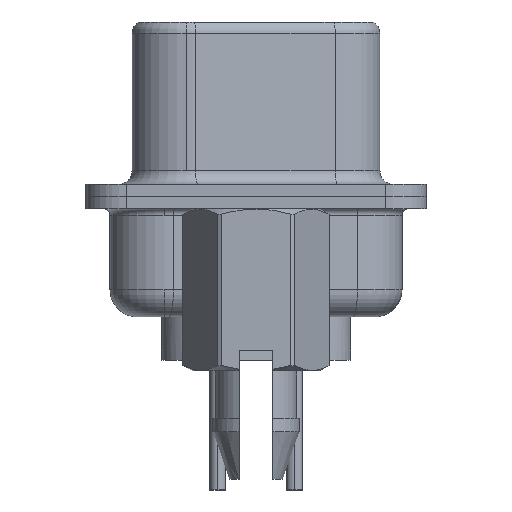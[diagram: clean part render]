
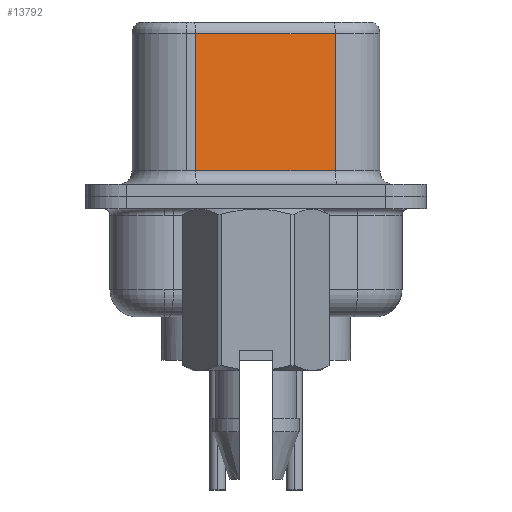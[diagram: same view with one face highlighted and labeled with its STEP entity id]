
A CAD part, left-side view. The second image highlights one B-rep face of the part: STEP entity #13792.
In plain terms, the highlighted planar face has unit normal (-0.985, -0.174, 0).
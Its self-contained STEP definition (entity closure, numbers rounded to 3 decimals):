
#142 = EDGE_CURVE ( 'NONE', #10876, #19702, #15350, .T. ) ;
#304 = LINE ( 'NONE', #4897, #16379 ) ;
#323 = VERTEX_POINT ( 'NONE', #346 ) ;
#346 = CARTESIAN_POINT ( 'NONE',  ( 4.575, -2.927, 6.02 ) ) ;
#371 = ORIENTED_EDGE ( 'NONE', *, *, #2547, .T. ) ;
#409 = DIRECTION ( 'NONE',  ( -0.174, 0.985, 0. ) ) ;
#1336 = ORIENTED_EDGE ( 'NONE', *, *, #4125, .T. ) ;
#1759 = CARTESIAN_POINT ( 'NONE',  ( 3.665, 2.233, 6.52 ) ) ;
#2231 = DIRECTION ( 'NONE',  ( 0.985, 0.174, 0. ) ) ;
#2373 = LINE ( 'NONE', #5272, #3210 ) ;
#2429 = PLANE ( 'NONE',  #13320 ) ;
#2547 = EDGE_CURVE ( 'NONE', #323, #10876, #304, .T. ) ;
#3210 = VECTOR ( 'NONE', #13266, 1000. ) ;
#3306 = VECTOR ( 'NONE', #12188, 1000. ) ;
#4047 = ORIENTED_EDGE ( 'NONE', *, *, #10381, .F. ) ;
#4125 = EDGE_CURVE ( 'NONE', #19702, #11844, #2373, .T. ) ;
#4897 = CARTESIAN_POINT ( 'NONE',  ( 4.575, -2.927, 6.02 ) ) ;
#5272 = CARTESIAN_POINT ( 'NONE',  ( 4.575, -2.927, 0.95 ) ) ;
#5894 = CARTESIAN_POINT ( 'NONE',  ( 4.575, -2.927, 6.52 ) ) ;
#5972 = VECTOR ( 'NONE', #7544, 1000. ) ;
#6085 = LINE ( 'NONE', #5894, #3306 ) ;
#7544 = DIRECTION ( 'NONE',  ( 0., 0., -1. ) ) ;
#8221 = CARTESIAN_POINT ( 'NONE',  ( 4.575, -2.927, 6.52 ) ) ;
#9478 = ORIENTED_EDGE ( 'NONE', *, *, #142, .T. ) ;
#10381 = EDGE_CURVE ( 'NONE', #323, #11844, #6085, .T. ) ;
#10876 = VERTEX_POINT ( 'NONE', #19478 ) ;
#10974 = EDGE_LOOP ( 'NONE', ( #4047, #371, #9478, #1336 ) ) ;
#11844 = VERTEX_POINT ( 'NONE', #18302 ) ;
#12188 = DIRECTION ( 'NONE',  ( 0., 0., -1. ) ) ;
#13266 = DIRECTION ( 'NONE',  ( 0.174, -0.985, 0. ) ) ;
#13320 = AXIS2_PLACEMENT_3D ( 'NONE', #8221, #2231, #15944 ) ;
#13792 = ADVANCED_FACE ( 'NONE', ( #19030 ), #2429, .F. ) ;
#15350 = LINE ( 'NONE', #1759, #5972 ) ;
#15944 = DIRECTION ( 'NONE',  ( -0.174, 0.985, 0. ) ) ;
#16379 = VECTOR ( 'NONE', #409, 1000. ) ;
#16994 = CARTESIAN_POINT ( 'NONE',  ( 3.665, 2.233, 0.95 ) ) ;
#18302 = CARTESIAN_POINT ( 'NONE',  ( 4.575, -2.927, 0.95 ) ) ;
#19030 = FACE_OUTER_BOUND ( 'NONE', #10974, .T. ) ;
#19478 = CARTESIAN_POINT ( 'NONE',  ( 3.665, 2.233, 6.02 ) ) ;
#19702 = VERTEX_POINT ( 'NONE', #16994 ) ;
